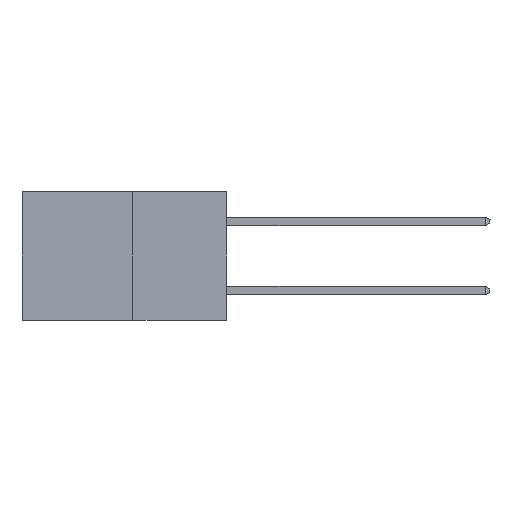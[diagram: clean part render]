
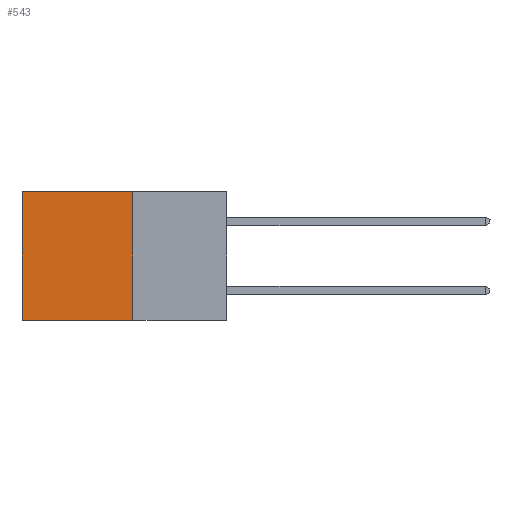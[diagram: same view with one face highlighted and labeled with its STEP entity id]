
A CAD part, left-side view. The second image highlights one B-rep face of the part: STEP entity #543.
In plain terms, the highlighted planar face has unit normal (-1, 0, 0).
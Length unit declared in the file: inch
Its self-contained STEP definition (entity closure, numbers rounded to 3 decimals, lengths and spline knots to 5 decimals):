
#424 = CARTESIAN_POINT ( 'NONE',  ( 0.277, 0.27, 0. ) ) ;
#543 = ADVANCED_FACE ( 'NONE', ( #7763 ), #10231, .F. ) ;
#583 = CARTESIAN_POINT ( 'NONE',  ( 0.277, 0.59, -0.37 ) ) ;
#2601 = VERTEX_POINT ( 'NONE', #13792 ) ;
#3012 = EDGE_LOOP ( 'NONE', ( #8385, #4111, #4263, #8800 ) ) ;
#3964 = LINE ( 'NONE', #16070, #15673 ) ;
#4111 = ORIENTED_EDGE ( 'NONE', *, *, #15290, .F. ) ;
#4263 = ORIENTED_EDGE ( 'NONE', *, *, #18291, .F. ) ;
#6343 = VECTOR ( 'NONE', #14343, 39.37008 ) ;
#6470 = CARTESIAN_POINT ( 'NONE',  ( 0.277, 0.27, -0.37 ) ) ;
#6825 = LINE ( 'NONE', #583, #6343 ) ;
#7763 = FACE_OUTER_BOUND ( 'NONE', #3012, .T. ) ;
#8123 = CARTESIAN_POINT ( 'NONE',  ( 0.277, 0.27, -0.37 ) ) ;
#8385 = ORIENTED_EDGE ( 'NONE', *, *, #13870, .T. ) ;
#8800 = ORIENTED_EDGE ( 'NONE', *, *, #17767, .T. ) ;
#10231 = PLANE ( 'NONE',  #10561 ) ;
#10561 = AXIS2_PLACEMENT_3D ( 'NONE', #12819, #12362, #10849 ) ;
#10849 = DIRECTION ( 'NONE',  ( 0., 0., -1. ) ) ;
#11179 = DIRECTION ( 'NONE',  ( 0., 0., -1. ) ) ;
#11184 = LINE ( 'NONE', #6470, #18698 ) ;
#11228 = VERTEX_POINT ( 'NONE', #424 ) ;
#11539 = DIRECTION ( 'NONE',  ( 0., 1., 0. ) ) ;
#11741 = CARTESIAN_POINT ( 'NONE',  ( 0.277, 0.59, -0.37 ) ) ;
#12362 = DIRECTION ( 'NONE',  ( 1., 0., 0. ) ) ;
#12819 = CARTESIAN_POINT ( 'NONE',  ( 0.277, 0.27, -0.37 ) ) ;
#12869 = VECTOR ( 'NONE', #17340, 39.37008 ) ;
#13335 = LINE ( 'NONE', #8123, #12869 ) ;
#13734 = VERTEX_POINT ( 'NONE', #15531 ) ;
#13792 = CARTESIAN_POINT ( 'NONE',  ( 0.277, 0.59, 0. ) ) ;
#13870 = EDGE_CURVE ( 'NONE', #2601, #16011, #6825, .T. ) ;
#14343 = DIRECTION ( 'NONE',  ( 0., 0., -1. ) ) ;
#15290 = EDGE_CURVE ( 'NONE', #13734, #16011, #13335, .T. ) ;
#15531 = CARTESIAN_POINT ( 'NONE',  ( 0.277, 0.27, -0.37 ) ) ;
#15673 = VECTOR ( 'NONE', #11539, 39.37008 ) ;
#16011 = VERTEX_POINT ( 'NONE', #11741 ) ;
#16070 = CARTESIAN_POINT ( 'NONE',  ( 0.277, 0.27, 0. ) ) ;
#17340 = DIRECTION ( 'NONE',  ( 0., 1., 0. ) ) ;
#17767 = EDGE_CURVE ( 'NONE', #11228, #2601, #3964, .T. ) ;
#18291 = EDGE_CURVE ( 'NONE', #11228, #13734, #11184, .T. ) ;
#18698 = VECTOR ( 'NONE', #11179, 39.37008 ) ;
